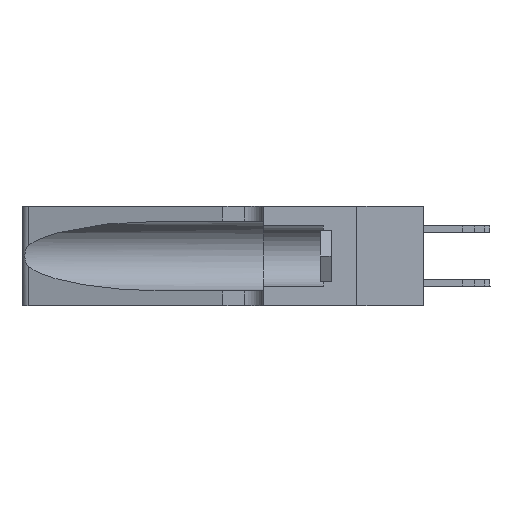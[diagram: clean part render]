
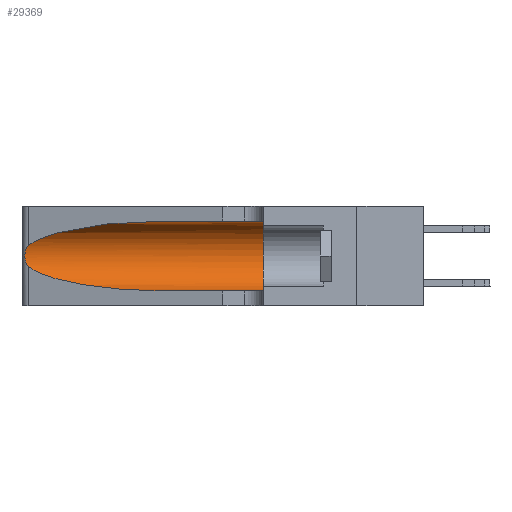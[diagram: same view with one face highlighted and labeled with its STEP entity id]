
A CAD part, left-side view. The second image highlights one B-rep face of the part: STEP entity #29369.
In plain terms, the highlighted cylindrical face has radius 3.308 mm (diameter 6.617 mm), a partial arc.
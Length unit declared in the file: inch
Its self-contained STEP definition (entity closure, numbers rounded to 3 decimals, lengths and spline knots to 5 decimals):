
#165 = ORIENTED_EDGE ( 'NONE', *, *, #25273, .T. ) ;
#994 = VERTEX_POINT ( 'NONE', #2005 ) ;
#1158 = CARTESIAN_POINT ( 'NONE',  ( 0.26017, 1.23833, 0.17102 ) ) ;
#1746 = CARTESIAN_POINT ( 'NONE',  ( 0.1305, 0.72297, 0.05475 ) ) ;
#2005 = CARTESIAN_POINT ( 'NONE',  ( 0.25487, 1.22718, 0.14631 ) ) ;
#2509 = CARTESIAN_POINT ( 'NONE',  ( 0.1305, 0.72297, 0.31525 ) ) ;
#3696 = CARTESIAN_POINT ( 'NONE',  ( 0.25555, 1.22993, 0.14849 ) ) ;
#3744 = ORIENTED_EDGE ( 'NONE', *, *, #25324, .T. ) ;
#3818 = CARTESIAN_POINT ( 'NONE',  ( 0.25787, 1.23484, 0.2124 ) ) ;
#4206 = EDGE_CURVE ( 'NONE', #9920, #13754, #6682, .T. ) ;
#4708 = CARTESIAN_POINT ( 'NONE',  ( 0.18966, 0.96281, 0.31525 ) ) ;
#4762 = CARTESIAN_POINT ( 'NONE',  ( 0.1305, 0.35, 0.185 ) ) ;
#4814 = CARTESIAN_POINT ( 'NONE',  ( 0.1305, 0.72297, 0.31525 ) ) ;
#6134 = CARTESIAN_POINT ( 'NONE',  ( 0.25789, 1.23486, 0.15765 ) ) ;
#6460 = DIRECTION ( 'NONE',  ( 0., -1., 0. ) ) ;
#6682 = CIRCLE ( 'NONE', #27403, 0.13025 ) ;
#6814 = FACE_OUTER_BOUND ( 'NONE', #10921, .T. ) ;
#7292 = DIRECTION ( 'NONE',  ( 0., 1., 0. ) ) ;
#7582 = CYLINDRICAL_SURFACE ( 'NONE', #9031, 0.13025 ) ;
#8564 = CARTESIAN_POINT ( 'NONE',  ( 0.25487, 1.22718, 0.14631 ) ) ;
#8939 = CARTESIAN_POINT ( 'NONE',  ( 0.18966, 0.96281, 0.05475 ) ) ;
#9031 = AXIS2_PLACEMENT_3D ( 'NONE', #16895, #6460, #23981 ) ;
#9810 = DIRECTION ( 'NONE',  ( 0., 0., 1. ) ) ;
#9920 = VERTEX_POINT ( 'NONE', #19110 ) ;
#10671 = ORIENTED_EDGE ( 'NONE', *, *, #24493, .F. ) ;
#10921 = EDGE_LOOP ( 'NONE', ( #16797, #17340, #165, #3744, #19981, #10671 ) ) ;
#11392 = CARTESIAN_POINT ( 'NONE',  ( 0.25555, 1.22994, 0.2215 ) ) ;
#11656 = CARTESIAN_POINT ( 'NONE',  ( 0.25487, 1.22718, 0.14631 ) ) ;
#11902 = VECTOR ( 'NONE', #28789, 39.37008 ) ;
#13490 = CARTESIAN_POINT ( 'NONE',  ( 0.25856, 1.23593, 0.16098 ) ) ;
#13600 = CARTESIAN_POINT ( 'NONE',  ( 0.25854, 1.2359, 0.20912 ) ) ;
#13713 = CARTESIAN_POINT ( 'NONE',  ( 0.25639, 1.23184, 0.21858 ) ) ;
#13754 = VERTEX_POINT ( 'NONE', #18099 ) ;
#16234 = CARTESIAN_POINT ( 'NONE',  ( 0.26018, 1.23835, 0.19895 ) ) ;
#16382 = VERTEX_POINT ( 'NONE', #30106 ) ;
#16797 = ORIENTED_EDGE ( 'NONE', *, *, #17417, .T. ) ;
#16895 = CARTESIAN_POINT ( 'NONE',  ( 0.1305, 1.61858, 0.185 ) ) ;
#17340 = ORIENTED_EDGE ( 'NONE', *, *, #29294, .T. ) ;
#17417 = EDGE_CURVE ( 'NONE', #20460, #16382, #24465, .T. ) ;
#18099 = CARTESIAN_POINT ( 'NONE',  ( 0.1305, 0.35, 0.05475 ) ) ;
#18636 =( BOUNDED_CURVE ( )  B_SPLINE_CURVE ( 3, ( #11656, #18884, #8939, #1746 ),
 .UNSPECIFIED., .F., .F. ) 
 B_SPLINE_CURVE_WITH_KNOTS ( ( 4, 4 ),
 ( 3.44316, 4.71239 ),
 .UNSPECIFIED. ) 
 CURVE ( )  GEOMETRIC_REPRESENTATION_ITEM ( )  RATIONAL_B_SPLINE_CURVE ( ( 1., 0.87, 0.87, 1. ) ) 
 REPRESENTATION_ITEM ( '' )  );
#18730 = CARTESIAN_POINT ( 'NONE',  ( 0.25639, 1.23186, 0.15144 ) ) ;
#18839 = CARTESIAN_POINT ( 'NONE',  ( 0.26075, 1.23896, 0.19203 ) ) ;
#18884 = CARTESIAN_POINT ( 'NONE',  ( 0.2373, 1.15595, 0.08982 ) ) ;
#18920 = DIRECTION ( 'NONE',  ( 0., -1., 0. ) ) ;
#19110 = CARTESIAN_POINT ( 'NONE',  ( 0.1305, 0.35, 0.31525 ) ) ;
#19981 = ORIENTED_EDGE ( 'NONE', *, *, #4206, .F. ) ;
#20460 = VERTEX_POINT ( 'NONE', #2509 ) ;
#20507 = LINE ( 'NONE', #21630, #11902 ) ;
#21369 = CARTESIAN_POINT ( 'NONE',  ( 0.26075, 1.23896, 0.178 ) ) ;
#21630 = CARTESIAN_POINT ( 'NONE',  ( 0.1305, 1.61858, 0.05475 ) ) ;
#22242 = CARTESIAN_POINT ( 'NONE',  ( 0.2373, 1.15595, 0.28018 ) ) ;
#23633 = CARTESIAN_POINT ( 'NONE',  ( 0.1305, 1.61858, 0.31525 ) ) ;
#23981 = DIRECTION ( 'NONE',  ( 0., 0., -1. ) ) ;
#24465 =( BOUNDED_CURVE ( )  B_SPLINE_CURVE ( 3, ( #4814, #4708, #22242, #32254 ),
 .UNSPECIFIED., .F., .F. ) 
 B_SPLINE_CURVE_WITH_KNOTS ( ( 4, 4 ),
 ( 1.5708, 2.84003 ),
 .UNSPECIFIED. ) 
 CURVE ( )  GEOMETRIC_REPRESENTATION_ITEM ( )  RATIONAL_B_SPLINE_CURVE ( ( 1., 0.87, 0.87, 1. ) ) 
 REPRESENTATION_ITEM ( '' )  );
#24493 = EDGE_CURVE ( 'NONE', #20460, #9920, #25638, .T. ) ;
#25273 = EDGE_CURVE ( 'NONE', #994, #29558, #18636, .T. ) ;
#25324 = EDGE_CURVE ( 'NONE', #29558, #13754, #20507, .T. ) ;
#25638 = LINE ( 'NONE', #23633, #31883 ) ;
#27017 = CARTESIAN_POINT ( 'NONE',  ( 0.1305, 0.72297, 0.05475 ) ) ;
#27403 = AXIS2_PLACEMENT_3D ( 'NONE', #4762, #7292, #9810 ) ;
#27837 = B_SPLINE_CURVE_WITH_KNOTS ( 'NONE', 3,
 ( #28634, #11392, #13713, #3818, #13600, #16234, #18839, #21369, #1158, #13490, #6134, #18730, #3696, #8564 ),
 .UNSPECIFIED., .F., .F.,
 ( 4, 2, 2, 2, 2, 2, 4 ),
 ( 0., 0.00027, 0.00053, 0.00107, 0.0016, 0.00187, 0.00214 ),
 .UNSPECIFIED. ) ;
#28634 = CARTESIAN_POINT ( 'NONE',  ( 0.25487, 1.22718, 0.22369 ) ) ;
#28789 = DIRECTION ( 'NONE',  ( 0., -1., 0. ) ) ;
#29294 = EDGE_CURVE ( 'NONE', #16382, #994, #27837, .T. ) ;
#29369 = ADVANCED_FACE ( 'NONE', ( #6814 ), #7582, .F. ) ;
#29558 = VERTEX_POINT ( 'NONE', #27017 ) ;
#30106 = CARTESIAN_POINT ( 'NONE',  ( 0.25487, 1.22718, 0.22369 ) ) ;
#31883 = VECTOR ( 'NONE', #18920, 39.37008 ) ;
#32254 = CARTESIAN_POINT ( 'NONE',  ( 0.25487, 1.22718, 0.22369 ) ) ;
